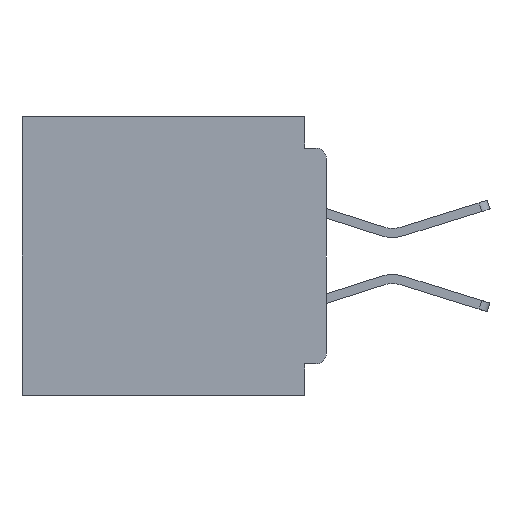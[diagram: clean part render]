
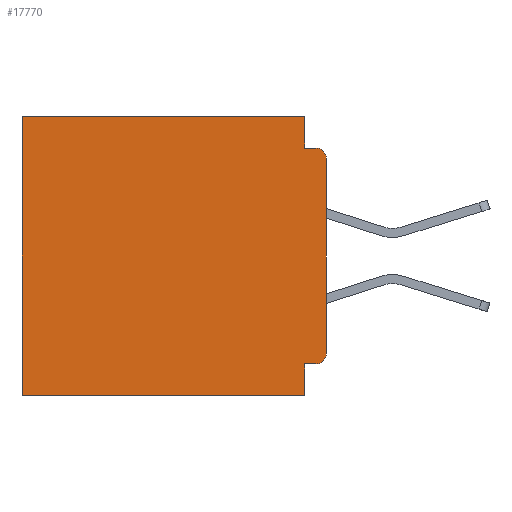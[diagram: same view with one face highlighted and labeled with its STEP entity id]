
A CAD part, left-side view. The second image highlights one B-rep face of the part: STEP entity #17770.
In plain terms, the highlighted planar face has unit normal (-1, 0, 0).
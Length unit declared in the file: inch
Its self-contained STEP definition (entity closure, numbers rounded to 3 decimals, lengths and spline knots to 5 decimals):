
#191 = LINE ( 'NONE', #11778, #22236 ) ;
#1889 = EDGE_CURVE ( 'NONE', #28340, #32247, #7788, .T. ) ;
#2998 = VERTEX_POINT ( 'NONE', #25041 ) ;
#3021 = DIRECTION ( 'NONE',  ( 0., 0., -1. ) ) ;
#3314 = AXIS2_PLACEMENT_3D ( 'NONE', #32417, #15607, #35151 ) ;
#3371 = VECTOR ( 'NONE', #23947, 39.37008 ) ;
#3599 = ORIENTED_EDGE ( 'NONE', *, *, #35037, .T. ) ;
#3645 = VECTOR ( 'NONE', #16005, 39.37008 ) ;
#3818 = LINE ( 'NONE', #15155, #33182 ) ;
#4235 = CARTESIAN_POINT ( 'NONE',  ( 0.3, 0.437, -0.4 ) ) ;
#4338 = ORIENTED_EDGE ( 'NONE', *, *, #26872, .F. ) ;
#5998 = CARTESIAN_POINT ( 'NONE',  ( 0.3, 0.031, -0.4 ) ) ;
#6433 = ORIENTED_EDGE ( 'NONE', *, *, #29290, .F. ) ;
#6691 = VERTEX_POINT ( 'NONE', #19268 ) ;
#6910 = FACE_OUTER_BOUND ( 'NONE', #17257, .T. ) ;
#7473 = PLANE ( 'NONE',  #15524 ) ;
#7788 = LINE ( 'NONE', #19522, #22104 ) ;
#8097 = CARTESIAN_POINT ( 'NONE',  ( 0.3, 0.031, -0.4 ) ) ;
#9533 = DIRECTION ( 'NONE',  ( -1., 0., 0. ) ) ;
#11054 = VERTEX_POINT ( 'NONE', #14505 ) ;
#11748 = AXIS2_PLACEMENT_3D ( 'NONE', #26588, #9533, #29464 ) ;
#11778 = CARTESIAN_POINT ( 'NONE',  ( 0.3, 0.437, -0.4 ) ) ;
#12267 = VECTOR ( 'NONE', #20524, 39.37008 ) ;
#12319 = LINE ( 'NONE', #24865, #18977 ) ;
#12962 = EDGE_CURVE ( 'NONE', #28340, #6691, #25087, .T. ) ;
#13125 = CARTESIAN_POINT ( 'NONE',  ( 0.3, 0., -0.4 ) ) ;
#13845 = ORIENTED_EDGE ( 'NONE', *, *, #24815, .F. ) ;
#14208 = LINE ( 'NONE', #5998, #20809 ) ;
#14367 = VERTEX_POINT ( 'NONE', #4235 ) ;
#14505 = CARTESIAN_POINT ( 'NONE',  ( 0.3, 0.031, 0. ) ) ;
#14719 = DIRECTION ( 'NONE',  ( 0., 0., -1. ) ) ;
#15155 = CARTESIAN_POINT ( 'NONE',  ( 0.3, 0.031, 0. ) ) ;
#15524 = AXIS2_PLACEMENT_3D ( 'NONE', #24549, #35724, #19006 ) ;
#15607 = DIRECTION ( 'NONE',  ( -1., 0., 0. ) ) ;
#16005 = DIRECTION ( 'NONE',  ( 0., 1., 0. ) ) ;
#17257 = EDGE_LOOP ( 'NONE', ( #20772, #21424, #4338, #21455, #28552, #3599, #6433, #13845, #31068, #33124 ) ) ;
#17348 = VERTEX_POINT ( 'NONE', #22735 ) ;
#17713 = CARTESIAN_POINT ( 'NONE',  ( 0.3, 0., -0.355 ) ) ;
#17770 = ADVANCED_FACE ( 'NONE', ( #6910 ), #7473, .F. ) ;
#18300 = VERTEX_POINT ( 'NONE', #26887 ) ;
#18713 = LINE ( 'NONE', #21136, #3371 ) ;
#18962 = LINE ( 'NONE', #13125, #3645 ) ;
#18977 = VECTOR ( 'NONE', #33177, 39.37008 ) ;
#19006 = DIRECTION ( 'NONE',  ( 0., 0., -1. ) ) ;
#19179 = EDGE_CURVE ( 'NONE', #11054, #21692, #12319, .T. ) ;
#19268 = CARTESIAN_POINT ( 'NONE',  ( 0.3, 0.015, -0.045 ) ) ;
#19522 = CARTESIAN_POINT ( 'NONE',  ( 0.3, 0., -0.4 ) ) ;
#20524 = DIRECTION ( 'NONE',  ( 0., 1., 0. ) ) ;
#20772 = ORIENTED_EDGE ( 'NONE', *, *, #1889, .F. ) ;
#20809 = VECTOR ( 'NONE', #3021, 39.37008 ) ;
#21136 = CARTESIAN_POINT ( 'NONE',  ( 0.3, 0., -0.045 ) ) ;
#21424 = ORIENTED_EDGE ( 'NONE', *, *, #12962, .T. ) ;
#21455 = ORIENTED_EDGE ( 'NONE', *, *, #23577, .F. ) ;
#21692 = VERTEX_POINT ( 'NONE', #34370 ) ;
#22104 = VECTOR ( 'NONE', #22527, 39.37008 ) ;
#22236 = VECTOR ( 'NONE', #14719, 39.37008 ) ;
#22527 = DIRECTION ( 'NONE',  ( 0., 0., -1. ) ) ;
#22735 = CARTESIAN_POINT ( 'NONE',  ( 0.3, 0.031, -0.355 ) ) ;
#23577 = EDGE_CURVE ( 'NONE', #11054, #2998, #3818, .T. ) ;
#23947 = DIRECTION ( 'NONE',  ( 0., -1., 0. ) ) ;
#24239 = CARTESIAN_POINT ( 'NONE',  ( 0.3, 0., -0.34 ) ) ;
#24549 = CARTESIAN_POINT ( 'NONE',  ( 0.3, 0., -0.4 ) ) ;
#24815 = EDGE_CURVE ( 'NONE', #17348, #25287, #14208, .T. ) ;
#24865 = CARTESIAN_POINT ( 'NONE',  ( 0.3, 0., 0. ) ) ;
#25041 = CARTESIAN_POINT ( 'NONE',  ( 0.3, 0.031, -0.045 ) ) ;
#25087 = CIRCLE ( 'NONE', #11748, 0.015 ) ;
#25287 = VERTEX_POINT ( 'NONE', #8097 ) ;
#26588 = CARTESIAN_POINT ( 'NONE',  ( 0.3, 0.015, -0.06 ) ) ;
#26872 = EDGE_CURVE ( 'NONE', #2998, #6691, #18713, .T. ) ;
#26887 = CARTESIAN_POINT ( 'NONE',  ( 0.3, 0.015, -0.355 ) ) ;
#27362 = LINE ( 'NONE', #17713, #12267 ) ;
#28340 = VERTEX_POINT ( 'NONE', #31468 ) ;
#28552 = ORIENTED_EDGE ( 'NONE', *, *, #19179, .T. ) ;
#29290 = EDGE_CURVE ( 'NONE', #25287, #14367, #18962, .T. ) ;
#29464 = DIRECTION ( 'NONE',  ( 0., 0., -1. ) ) ;
#29708 = EDGE_CURVE ( 'NONE', #18300, #17348, #27362, .T. ) ;
#31068 = ORIENTED_EDGE ( 'NONE', *, *, #29708, .F. ) ;
#31468 = CARTESIAN_POINT ( 'NONE',  ( 0.3, 0., -0.06 ) ) ;
#32247 = VERTEX_POINT ( 'NONE', #24239 ) ;
#32376 = CIRCLE ( 'NONE', #3314, 0.015 ) ;
#32417 = CARTESIAN_POINT ( 'NONE',  ( 0.3, 0.015, -0.34 ) ) ;
#33124 = ORIENTED_EDGE ( 'NONE', *, *, #34570, .T. ) ;
#33177 = DIRECTION ( 'NONE',  ( 0., 1., 0. ) ) ;
#33182 = VECTOR ( 'NONE', #34723, 39.37008 ) ;
#34370 = CARTESIAN_POINT ( 'NONE',  ( 0.3, 0.437, 0. ) ) ;
#34570 = EDGE_CURVE ( 'NONE', #18300, #32247, #32376, .T. ) ;
#34723 = DIRECTION ( 'NONE',  ( 0., 0., -1. ) ) ;
#35037 = EDGE_CURVE ( 'NONE', #21692, #14367, #191, .T. ) ;
#35151 = DIRECTION ( 'NONE',  ( 0., 0., -1. ) ) ;
#35724 = DIRECTION ( 'NONE',  ( 1., 0., 0. ) ) ;
